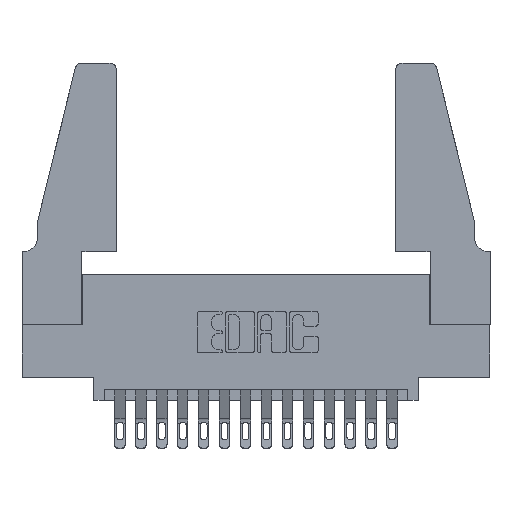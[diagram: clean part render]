
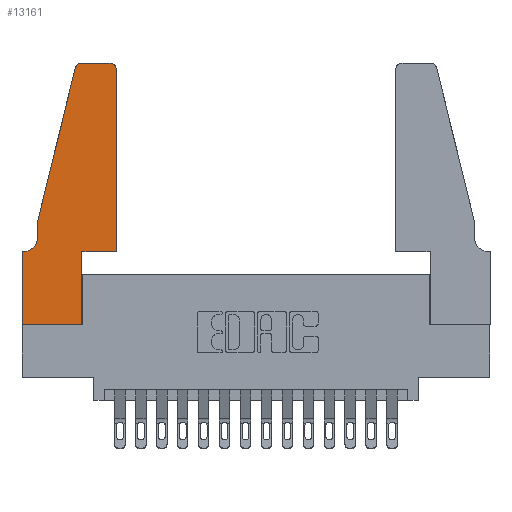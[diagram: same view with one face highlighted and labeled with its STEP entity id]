
A CAD part, top view. The second image highlights one B-rep face of the part: STEP entity #13161.
In plain terms, the highlighted planar face has unit normal (0, 0, 1).
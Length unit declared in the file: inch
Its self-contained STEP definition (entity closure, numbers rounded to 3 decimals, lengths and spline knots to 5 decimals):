
#64 = CARTESIAN_POINT ( 'NONE',  ( 0.2605, 1.25, 0.37 ) ) ;
#445 = EDGE_CURVE ( 'NONE', #8895, #7503, #5725, .T. ) ;
#578 = CARTESIAN_POINT ( 'NONE',  ( 0., 0., 0.37 ) ) ;
#788 = CIRCLE ( 'NONE', #16249, 0.03 ) ;
#882 = ORIENTED_EDGE ( 'NONE', *, *, #11972, .T. ) ;
#916 = ORIENTED_EDGE ( 'NONE', *, *, #3643, .T. ) ;
#1166 = DIRECTION ( 'NONE',  ( 0., 0., 1. ) ) ;
#1207 = CARTESIAN_POINT ( 'NONE',  ( 0.284, 1.25, 0.37 ) ) ;
#1447 = VECTOR ( 'NONE', #14443, 39.37008 ) ;
#1575 = EDGE_CURVE ( 'NONE', #17287, #14014, #9698, .T. ) ;
#1866 = LINE ( 'NONE', #15776, #1447 ) ;
#2083 = ORIENTED_EDGE ( 'NONE', *, *, #445, .T. ) ;
#2156 = VECTOR ( 'NONE', #4653, 39.37008 ) ;
#2233 = ORIENTED_EDGE ( 'NONE', *, *, #7841, .T. ) ;
#2339 = VECTOR ( 'NONE', #12684, 39.37008 ) ;
#2507 = AXIS2_PLACEMENT_3D ( 'NONE', #4895, #14267, #6228 ) ;
#2558 = LINE ( 'NONE', #64, #9271 ) ;
#2765 = CARTESIAN_POINT ( 'NONE',  ( 0.4505, 1.22, 0.37 ) ) ;
#2800 = DIRECTION ( 'NONE',  ( -1., 0., 0. ) ) ;
#2873 = CARTESIAN_POINT ( 'NONE',  ( 0.0755, 0.35, 0.37 ) ) ;
#2931 = DIRECTION ( 'NONE',  ( -1., 0., 0. ) ) ;
#2932 = VERTEX_POINT ( 'NONE', #17012 ) ;
#2974 = CARTESIAN_POINT ( 'NONE',  ( 0.2865, 0., 0.37 ) ) ;
#3277 = CARTESIAN_POINT ( 'NONE',  ( 0.4505, 0.35, 0.37 ) ) ;
#3320 = EDGE_CURVE ( 'NONE', #9896, #17287, #11797, .T. ) ;
#3643 = EDGE_CURVE ( 'NONE', #7503, #10708, #788, .T. ) ;
#4419 = CARTESIAN_POINT ( 'NONE',  ( 0.4505, 0.35, 0.37 ) ) ;
#4653 = DIRECTION ( 'NONE',  ( 0., 1., 0. ) ) ;
#4895 = CARTESIAN_POINT ( 'NONE',  ( 0.0055, 0.42, 0.37 ) ) ;
#5079 = CARTESIAN_POINT ( 'NONE',  ( 0.284, 1.22, 0.37 ) ) ;
#5180 = EDGE_CURVE ( 'NONE', #14014, #5381, #10855, .T. ) ;
#5295 = CARTESIAN_POINT ( 'NONE',  ( 0.4205, 1.25, 0.37 ) ) ;
#5381 = VERTEX_POINT ( 'NONE', #6344 ) ;
#5647 = CARTESIAN_POINT ( 'NONE',  ( 0., 0., 0.37 ) ) ;
#5695 = CARTESIAN_POINT ( 'NONE',  ( 0.4505, 0.35, 0.37 ) ) ;
#5725 = LINE ( 'NONE', #4419, #2156 ) ;
#5826 = AXIS2_PLACEMENT_3D ( 'NONE', #5079, #14459, #6428 ) ;
#5881 = CARTESIAN_POINT ( 'NONE',  ( 0.2865, 0.35, 0.37 ) ) ;
#6228 = DIRECTION ( 'NONE',  ( -1., 0., 0. ) ) ;
#6344 = CARTESIAN_POINT ( 'NONE',  ( 0.2865, 0.35, 0.37 ) ) ;
#6428 = DIRECTION ( 'NONE',  ( 1., 0., 0. ) ) ;
#6683 = VERTEX_POINT ( 'NONE', #7851 ) ;
#7336 = DIRECTION ( 'NONE',  ( -0.239, -0.971, 0. ) ) ;
#7360 = ORIENTED_EDGE ( 'NONE', *, *, #13353, .T. ) ;
#7503 = VERTEX_POINT ( 'NONE', #2765 ) ;
#7708 = CARTESIAN_POINT ( 'NONE',  ( 0.4205, 1.22, 0.37 ) ) ;
#7841 = EDGE_CURVE ( 'NONE', #2932, #6683, #14938, .T. ) ;
#7851 = CARTESIAN_POINT ( 'NONE',  ( 0.0755, 0.5, 0.37 ) ) ;
#8174 = VECTOR ( 'NONE', #8351, 39.37008 ) ;
#8351 = DIRECTION ( 'NONE',  ( 0., -1., 0. ) ) ;
#8567 = EDGE_CURVE ( 'NONE', #16782, #9583, #10310, .T. ) ;
#8683 = ORIENTED_EDGE ( 'NONE', *, *, #8567, .T. ) ;
#8895 = VERTEX_POINT ( 'NONE', #5695 ) ;
#8976 = CIRCLE ( 'NONE', #5826, 0.03 ) ;
#8978 = AXIS2_PLACEMENT_3D ( 'NONE', #9216, #1166, #10579 ) ;
#9044 = DIRECTION ( 'NONE',  ( 1., 0., 0. ) ) ;
#9072 = CARTESIAN_POINT ( 'NONE',  ( 0., 0.35, 0.37 ) ) ;
#9173 = ORIENTED_EDGE ( 'NONE', *, *, #1575, .T. ) ;
#9216 = CARTESIAN_POINT ( 'NONE',  ( 0., 0.35, 0.37 ) ) ;
#9271 = VECTOR ( 'NONE', #2800, 39.37008 ) ;
#9583 = VERTEX_POINT ( 'NONE', #12582 ) ;
#9698 = LINE ( 'NONE', #10606, #13304 ) ;
#9896 = VERTEX_POINT ( 'NONE', #9072 ) ;
#10310 = CIRCLE ( 'NONE', #2507, 0.07 ) ;
#10380 = DIRECTION ( 'NONE',  ( 1., 0., 0. ) ) ;
#10579 = DIRECTION ( 'NONE',  ( 1., 0., 0. ) ) ;
#10606 = CARTESIAN_POINT ( 'NONE',  ( 0., 0., 0.37 ) ) ;
#10708 = VERTEX_POINT ( 'NONE', #5295 ) ;
#10847 = ORIENTED_EDGE ( 'NONE', *, *, #13095, .T. ) ;
#10855 = LINE ( 'NONE', #5881, #13984 ) ;
#10939 = FACE_OUTER_BOUND ( 'NONE', #12422, .T. ) ;
#11139 = VECTOR ( 'NONE', #2931, 39.37008 ) ;
#11371 = VERTEX_POINT ( 'NONE', #1207 ) ;
#11429 = VECTOR ( 'NONE', #7336, 39.37008 ) ;
#11797 = LINE ( 'NONE', #5647, #8174 ) ;
#11972 = EDGE_CURVE ( 'NONE', #10708, #11371, #2558, .T. ) ;
#12170 = EDGE_CURVE ( 'NONE', #5381, #8895, #13896, .T. ) ;
#12422 = EDGE_LOOP ( 'NONE', ( #882, #14852, #2233, #10847, #8683, #7360, #16318, #9173, #14757, #14698, #2083, #916 ) ) ;
#12582 = CARTESIAN_POINT ( 'NONE',  ( 0.0055, 0.35, 0.37 ) ) ;
#12684 = DIRECTION ( 'NONE',  ( 1., 0., 0. ) ) ;
#13095 = EDGE_CURVE ( 'NONE', #6683, #16782, #1866, .T. ) ;
#13161 = ADVANCED_FACE ( 'NONE', ( #10939 ), #13238, .T. ) ;
#13238 = PLANE ( 'NONE',  #8978 ) ;
#13304 = VECTOR ( 'NONE', #10380, 39.37008 ) ;
#13353 = EDGE_CURVE ( 'NONE', #9583, #9896, #14675, .T. ) ;
#13896 = LINE ( 'NONE', #3277, #2339 ) ;
#13934 = DIRECTION ( 'NONE',  ( 0., 1., 0. ) ) ;
#13984 = VECTOR ( 'NONE', #13934, 39.37008 ) ;
#14014 = VERTEX_POINT ( 'NONE', #2974 ) ;
#14267 = DIRECTION ( 'NONE',  ( 0., 0., -1. ) ) ;
#14399 = EDGE_CURVE ( 'NONE', #11371, #2932, #8976, .T. ) ;
#14443 = DIRECTION ( 'NONE',  ( 0., -1., 0. ) ) ;
#14459 = DIRECTION ( 'NONE',  ( 0., 0., 1. ) ) ;
#14675 = LINE ( 'NONE', #2873, #11139 ) ;
#14698 = ORIENTED_EDGE ( 'NONE', *, *, #12170, .T. ) ;
#14757 = ORIENTED_EDGE ( 'NONE', *, *, #5180, .T. ) ;
#14852 = ORIENTED_EDGE ( 'NONE', *, *, #14399, .T. ) ;
#14938 = LINE ( 'NONE', #15470, #11429 ) ;
#15470 = CARTESIAN_POINT ( 'NONE',  ( 0.0755, 0.5, 0.37 ) ) ;
#15776 = CARTESIAN_POINT ( 'NONE',  ( 0.0755, 0.5, 0.37 ) ) ;
#16249 = AXIS2_PLACEMENT_3D ( 'NONE', #7708, #17052, #9044 ) ;
#16318 = ORIENTED_EDGE ( 'NONE', *, *, #3320, .T. ) ;
#16782 = VERTEX_POINT ( 'NONE', #17032 ) ;
#17012 = CARTESIAN_POINT ( 'NONE',  ( 0.25487, 1.22718, 0.37 ) ) ;
#17032 = CARTESIAN_POINT ( 'NONE',  ( 0.0755, 0.42, 0.37 ) ) ;
#17052 = DIRECTION ( 'NONE',  ( 0., 0., 1. ) ) ;
#17287 = VERTEX_POINT ( 'NONE', #578 ) ;
